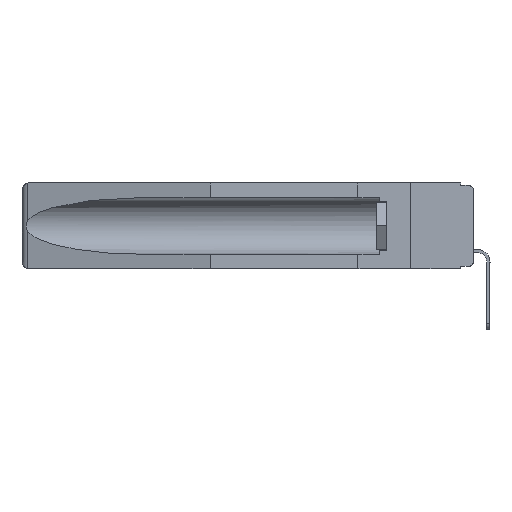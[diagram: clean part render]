
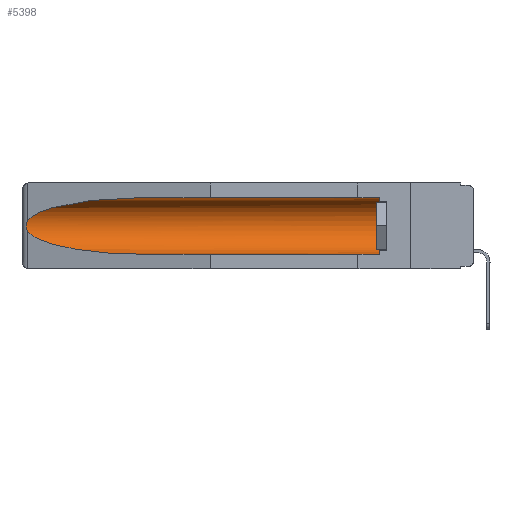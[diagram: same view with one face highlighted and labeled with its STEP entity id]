
A CAD part, left-side view. The second image highlights one B-rep face of the part: STEP entity #5398.
In plain terms, the highlighted cylindrical face has radius 2.857 mm (diameter 5.715 mm), a partial arc.
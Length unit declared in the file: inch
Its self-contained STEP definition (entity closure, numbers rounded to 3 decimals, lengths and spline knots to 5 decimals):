
#28 = CIRCLE ( 'NONE', #9083, 0.1125 ) ;
#441 = CARTESIAN_POINT ( 'NONE',  ( 0.155, 0.126, -0.1715 ) ) ;
#705 =( BOUNDED_CURVE ( )  B_SPLINE_CURVE ( 3, ( #17198, #15289, #15732, #10518 ),
 .UNSPECIFIED., .F., .F. ) 
 B_SPLINE_CURVE_WITH_KNOTS ( ( 4, 4 ),
 ( 4.71239, 6.08839 ),
 .UNSPECIFIED. ) 
 CURVE ( )  GEOMETRIC_REPRESENTATION_ITEM ( )  RATIONAL_B_SPLINE_CURVE ( ( 1., 0.848, 0.848, 1. ) ) 
 REPRESENTATION_ITEM ( '' )  );
#861 = LINE ( 'NONE', #19802, #13269 ) ;
#864 = EDGE_CURVE ( 'NONE', #14825, #5829, #28, .T. ) ;
#2390 = EDGE_CURVE ( 'NONE', #4413, #3299, #705, .T. ) ;
#3200 = ORIENTED_EDGE ( 'NONE', *, *, #10199, .T. ) ;
#3299 = VERTEX_POINT ( 'NONE', #7754 ) ;
#3331 = CARTESIAN_POINT ( 'NONE',  ( 0.155, 1.07973, -0.284 ) ) ;
#3408 = CARTESIAN_POINT ( 'NONE',  ( 0.26537, 1.52718, -0.14972 ) ) ;
#3761 = DIRECTION ( 'NONE',  ( 0., 0., 1. ) ) ;
#4343 = VERTEX_POINT ( 'NONE', #6238 ) ;
#4413 = VERTEX_POINT ( 'NONE', #18248 ) ;
#4438 = CARTESIAN_POINT ( 'NONE',  ( 0.155, 0.126, -0.059 ) ) ;
#5020 = CARTESIAN_POINT ( 'NONE',  ( 0.26537, 1.52718, -0.19328 ) ) ;
#5398 = ADVANCED_FACE ( 'NONE', ( #12163 ), #12269, .F. ) ;
#5433 = DIRECTION ( 'NONE',  ( 0., -1., 0. ) ) ;
#5552 = CARTESIAN_POINT ( 'NONE',  ( 0.26655, 1.53094, -0.18657 ) ) ;
#5829 = VERTEX_POINT ( 'NONE', #4438 ) ;
#6238 = CARTESIAN_POINT ( 'NONE',  ( 0.26537, 1.52718, -0.19328 ) ) ;
#6617 = VERTEX_POINT ( 'NONE', #11193 ) ;
#7239 = CARTESIAN_POINT ( 'NONE',  ( 0.26654, 1.53092, -0.15636 ) ) ;
#7567 = DIRECTION ( 'NONE',  ( 0., 0., 1. ) ) ;
#7754 = CARTESIAN_POINT ( 'NONE',  ( 0.26537, 1.52718, -0.14972 ) ) ;
#7763 = DIRECTION ( 'NONE',  ( 0., 1., 0. ) ) ;
#8185 = EDGE_CURVE ( 'NONE', #5829, #4413, #10830, .T. ) ;
#8556 = CARTESIAN_POINT ( 'NONE',  ( 0.155, -0.30754, -0.059 ) ) ;
#8840 = CARTESIAN_POINT ( 'NONE',  ( 0.2675, 1.53308, -0.17534 ) ) ;
#9083 = AXIS2_PLACEMENT_3D ( 'NONE', #441, #5433, #7567 ) ;
#10199 = EDGE_CURVE ( 'NONE', #3299, #4343, #16606, .T. ) ;
#10234 = DIRECTION ( 'NONE',  ( 0., 1., 0. ) ) ;
#10447 = CARTESIAN_POINT ( 'NONE',  ( 0.155, -0.30754, -0.1715 ) ) ;
#10518 = CARTESIAN_POINT ( 'NONE',  ( 0.26537, 1.52718, -0.14972 ) ) ;
#10830 = LINE ( 'NONE', #8556, #15485 ) ;
#11193 = CARTESIAN_POINT ( 'NONE',  ( 0.155, 1.07973, -0.284 ) ) ;
#11839 = CARTESIAN_POINT ( 'NONE',  ( 0.25451, 1.48313, -0.24835 ) ) ;
#11960 = CARTESIAN_POINT ( 'NONE',  ( 0.21114, 1.30732, -0.284 ) ) ;
#12163 = FACE_OUTER_BOUND ( 'NONE', #14226, .T. ) ;
#12269 = CYLINDRICAL_SURFACE ( 'NONE', #20406, 0.1125 ) ;
#13269 = VECTOR ( 'NONE', #7763, 39.37008 ) ;
#13548 = ORIENTED_EDGE ( 'NONE', *, *, #17852, .T. ) ;
#13739 = CARTESIAN_POINT ( 'NONE',  ( 0.26597, 1.5296, -0.19026 ) ) ;
#13962 = CARTESIAN_POINT ( 'NONE',  ( 0.155, 0.126, -0.284 ) ) ;
#14188 = CARTESIAN_POINT ( 'NONE',  ( 0.2675, 1.53308, -0.16763 ) ) ;
#14225 = ORIENTED_EDGE ( 'NONE', *, *, #864, .T. ) ;
#14226 = EDGE_LOOP ( 'NONE', ( #18460, #3200, #13548, #14670, #14225, #21486 ) ) ;
#14670 = ORIENTED_EDGE ( 'NONE', *, *, #16047, .F. ) ;
#14825 = VERTEX_POINT ( 'NONE', #13962 ) ;
#15289 = CARTESIAN_POINT ( 'NONE',  ( 0.21114, 1.30732, -0.059 ) ) ;
#15472 = DIRECTION ( 'NONE',  ( 0., 1., 0. ) ) ;
#15485 = VECTOR ( 'NONE', #15472, 39.37008 ) ;
#15732 = CARTESIAN_POINT ( 'NONE',  ( 0.25451, 1.48313, -0.09465 ) ) ;
#16047 = EDGE_CURVE ( 'NONE', #14825, #6617, #861, .T. ) ;
#16606 = B_SPLINE_CURVE_WITH_KNOTS ( 'NONE', 3,
 ( #3408, #17345, #7239, #20750, #14188, #8840, #22343, #5552, #13739, #17233 ),
 .UNSPECIFIED., .F., .F.,
 ( 4, 2, 2, 2, 4 ),
 ( 0., 0.00029, 0.00058, 0.00087, 0.00117 ),
 .UNSPECIFIED. ) ;
#17198 = CARTESIAN_POINT ( 'NONE',  ( 0.155, 1.07973, -0.059 ) ) ;
#17233 = CARTESIAN_POINT ( 'NONE',  ( 0.26537, 1.52718, -0.19328 ) ) ;
#17345 = CARTESIAN_POINT ( 'NONE',  ( 0.26597, 1.52961, -0.15275 ) ) ;
#17852 = EDGE_CURVE ( 'NONE', #4343, #6617, #22425, .T. ) ;
#18248 = CARTESIAN_POINT ( 'NONE',  ( 0.155, 1.07973, -0.059 ) ) ;
#18460 = ORIENTED_EDGE ( 'NONE', *, *, #2390, .T. ) ;
#19802 = CARTESIAN_POINT ( 'NONE',  ( 0.155, -0.30754, -0.284 ) ) ;
#20406 = AXIS2_PLACEMENT_3D ( 'NONE', #10447, #10234, #3761 ) ;
#20750 = CARTESIAN_POINT ( 'NONE',  ( 0.2673, 1.5327, -0.16383 ) ) ;
#21486 = ORIENTED_EDGE ( 'NONE', *, *, #8185, .T. ) ;
#22343 = CARTESIAN_POINT ( 'NONE',  ( 0.2673, 1.53269, -0.17917 ) ) ;
#22425 =( BOUNDED_CURVE ( )  B_SPLINE_CURVE ( 3, ( #5020, #11839, #11960, #3331 ),
 .UNSPECIFIED., .F., .F. ) 
 B_SPLINE_CURVE_WITH_KNOTS ( ( 4, 4 ),
 ( 0.1948, 1.5708 ),
 .UNSPECIFIED. ) 
 CURVE ( )  GEOMETRIC_REPRESENTATION_ITEM ( )  RATIONAL_B_SPLINE_CURVE ( ( 1., 0.848, 0.848, 1. ) ) 
 REPRESENTATION_ITEM ( '' )  );
